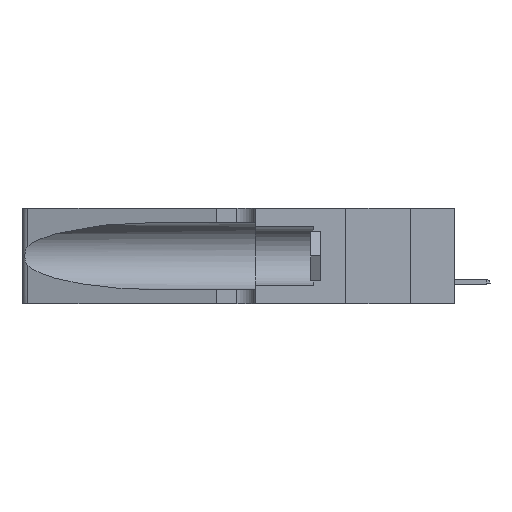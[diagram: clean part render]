
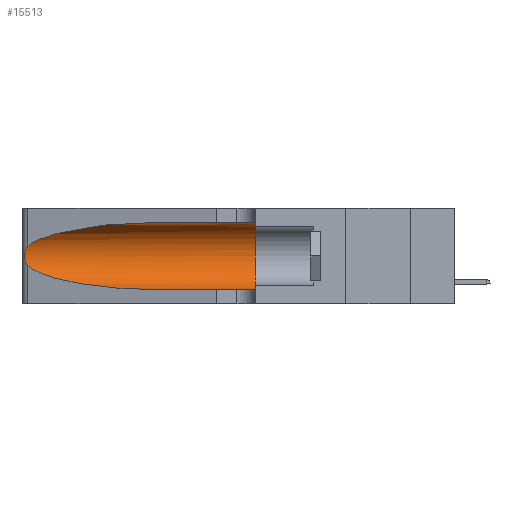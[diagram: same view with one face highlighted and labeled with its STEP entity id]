
A CAD part, left-side view. The second image highlights one B-rep face of the part: STEP entity #15513.
In plain terms, the highlighted cylindrical face has radius 3.308 mm (diameter 6.617 mm), a partial arc.
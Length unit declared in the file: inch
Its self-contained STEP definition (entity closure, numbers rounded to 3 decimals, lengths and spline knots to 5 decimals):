
#500 = CARTESIAN_POINT ( 'NONE',  ( 0.26018, 1.23835, 0.19895 ) ) ;
#1418 = VERTEX_POINT ( 'NONE', #24342 ) ;
#1615 = LINE ( 'NONE', #13818, #26982 ) ;
#2284 = EDGE_CURVE ( 'NONE', #27723, #1418, #1615, .T. ) ;
#5105 = CARTESIAN_POINT ( 'NONE',  ( 0.18966, 0.96281, 0.31525 ) ) ;
#5644 = VERTEX_POINT ( 'NONE', #38142 ) ;
#6279 = DIRECTION ( 'NONE',  ( 0., 1., 0. ) ) ;
#6294 = VERTEX_POINT ( 'NONE', #31980 ) ;
#6656 = AXIS2_PLACEMENT_3D ( 'NONE', #29112, #31883, #32481 ) ;
#7006 = CARTESIAN_POINT ( 'NONE',  ( 0.25856, 1.23593, 0.16098 ) ) ;
#7173 = DIRECTION ( 'NONE',  ( 0., -1., 0. ) ) ;
#7711 = ORIENTED_EDGE ( 'NONE', *, *, #32891, .T. ) ;
#7900 = FACE_OUTER_BOUND ( 'NONE', #38821, .T. ) ;
#8730 = CARTESIAN_POINT ( 'NONE',  ( 0.25487, 1.22718, 0.14631 ) ) ;
#9931 = CARTESIAN_POINT ( 'NONE',  ( 0.26017, 1.23833, 0.17102 ) ) ;
#10299 = CARTESIAN_POINT ( 'NONE',  ( 0.1305, 1.61858, 0.05475 ) ) ;
#11039 = CARTESIAN_POINT ( 'NONE',  ( 0.1305, 0.72297, 0.31525 ) ) ;
#11617 = CARTESIAN_POINT ( 'NONE',  ( 0.1305, 0.72297, 0.05475 ) ) ;
#12183 = CARTESIAN_POINT ( 'NONE',  ( 0.1305, 0.35, 0.185 ) ) ;
#12521 = CARTESIAN_POINT ( 'NONE',  ( 0.25555, 1.22993, 0.14849 ) ) ;
#12930 = EDGE_CURVE ( 'NONE', #1418, #5644, #25940, .T. ) ;
#13389 = CARTESIAN_POINT ( 'NONE',  ( 0.1305, 0.72297, 0.05475 ) ) ;
#13818 = CARTESIAN_POINT ( 'NONE',  ( 0.1305, 1.61858, 0.31525 ) ) ;
#14164 = CARTESIAN_POINT ( 'NONE',  ( 0.2373, 1.15595, 0.28018 ) ) ;
#15513 = ADVANCED_FACE ( 'NONE', ( #7900 ), #32087, .F. ) ;
#16052 = CARTESIAN_POINT ( 'NONE',  ( 0.25639, 1.23186, 0.15144 ) ) ;
#17863 = VECTOR ( 'NONE', #7173, 39.37008 ) ;
#18052 = EDGE_CURVE ( 'NONE', #6294, #21579, #19097, .T. ) ;
#18877 = CARTESIAN_POINT ( 'NONE',  ( 0.25487, 1.22718, 0.14631 ) ) ;
#18974 = CARTESIAN_POINT ( 'NONE',  ( 0.26075, 1.23896, 0.19203 ) ) ;
#19097 = B_SPLINE_CURVE_WITH_KNOTS ( 'NONE', 3,
 ( #31183, #24871, #24491, #30425, #36910, #500, #18974, #33961, #9931, #7006, #30990, #16052, #12521, #8730 ),
 .UNSPECIFIED., .F., .F.,
 ( 4, 2, 2, 2, 2, 2, 4 ),
 ( 0., 0.00027, 0.00053, 0.00107, 0.0016, 0.00187, 0.00214 ),
 .UNSPECIFIED. ) ;
#19181 = ORIENTED_EDGE ( 'NONE', *, *, #31482, .T. ) ;
#19891 = DIRECTION ( 'NONE',  ( 0., -1., 0. ) ) ;
#19926 = ORIENTED_EDGE ( 'NONE', *, *, #37539, .T. ) ;
#20940 =( BOUNDED_CURVE ( )  B_SPLINE_CURVE ( 3, ( #18877, #30886, #30695, #13389 ),
 .UNSPECIFIED., .F., .T. ) 
 B_SPLINE_CURVE_WITH_KNOTS ( ( 4, 4 ),
 ( 3.44316, 4.71239 ),
 .UNSPECIFIED. ) 
 CURVE ( )  GEOMETRIC_REPRESENTATION_ITEM ( )  RATIONAL_B_SPLINE_CURVE ( ( 1., 0.87, 0.87, 1. ) ) 
 REPRESENTATION_ITEM ( '' )  );
#21579 = VERTEX_POINT ( 'NONE', #32590 ) ;
#21766 = ORIENTED_EDGE ( 'NONE', *, *, #12930, .F. ) ;
#24342 = CARTESIAN_POINT ( 'NONE',  ( 0.1305, 0.35, 0.31525 ) ) ;
#24491 = CARTESIAN_POINT ( 'NONE',  ( 0.25639, 1.23184, 0.21858 ) ) ;
#24871 = CARTESIAN_POINT ( 'NONE',  ( 0.25555, 1.22994, 0.2215 ) ) ;
#24913 = DIRECTION ( 'NONE',  ( 0., 0., 1. ) ) ;
#24956 =( BOUNDED_CURVE ( )  B_SPLINE_CURVE ( 3, ( #28896, #5105, #14164, #38382 ),
 .UNSPECIFIED., .F., .F. ) 
 B_SPLINE_CURVE_WITH_KNOTS ( ( 4, 4 ),
 ( 1.5708, 2.84003 ),
 .UNSPECIFIED. ) 
 CURVE ( )  GEOMETRIC_REPRESENTATION_ITEM ( )  RATIONAL_B_SPLINE_CURVE ( ( 1., 0.87, 0.87, 1. ) ) 
 REPRESENTATION_ITEM ( '' )  );
#25609 = LINE ( 'NONE', #10299, #17863 ) ;
#25940 = CIRCLE ( 'NONE', #38585, 0.13025 ) ;
#26519 = ORIENTED_EDGE ( 'NONE', *, *, #18052, .T. ) ;
#26593 = ORIENTED_EDGE ( 'NONE', *, *, #2284, .F. ) ;
#26982 = VECTOR ( 'NONE', #19891, 39.37008 ) ;
#27723 = VERTEX_POINT ( 'NONE', #11039 ) ;
#28896 = CARTESIAN_POINT ( 'NONE',  ( 0.1305, 0.72297, 0.31525 ) ) ;
#29112 = CARTESIAN_POINT ( 'NONE',  ( 0.1305, 1.61858, 0.185 ) ) ;
#30425 = CARTESIAN_POINT ( 'NONE',  ( 0.25787, 1.23484, 0.2124 ) ) ;
#30695 = CARTESIAN_POINT ( 'NONE',  ( 0.18966, 0.96281, 0.05475 ) ) ;
#30886 = CARTESIAN_POINT ( 'NONE',  ( 0.2373, 1.15595, 0.08982 ) ) ;
#30990 = CARTESIAN_POINT ( 'NONE',  ( 0.25789, 1.23486, 0.15765 ) ) ;
#31183 = CARTESIAN_POINT ( 'NONE',  ( 0.25487, 1.22718, 0.22369 ) ) ;
#31482 = EDGE_CURVE ( 'NONE', #21579, #34091, #20940, .T. ) ;
#31883 = DIRECTION ( 'NONE',  ( 0., -1., 0. ) ) ;
#31980 = CARTESIAN_POINT ( 'NONE',  ( 0.25487, 1.22718, 0.22369 ) ) ;
#32087 = CYLINDRICAL_SURFACE ( 'NONE', #6656, 0.13025 ) ;
#32481 = DIRECTION ( 'NONE',  ( 0., 0., -1. ) ) ;
#32590 = CARTESIAN_POINT ( 'NONE',  ( 0.25487, 1.22718, 0.14631 ) ) ;
#32891 = EDGE_CURVE ( 'NONE', #27723, #6294, #24956, .T. ) ;
#33961 = CARTESIAN_POINT ( 'NONE',  ( 0.26075, 1.23896, 0.178 ) ) ;
#34091 = VERTEX_POINT ( 'NONE', #11617 ) ;
#36910 = CARTESIAN_POINT ( 'NONE',  ( 0.25854, 1.2359, 0.20912 ) ) ;
#37539 = EDGE_CURVE ( 'NONE', #34091, #5644, #25609, .T. ) ;
#38142 = CARTESIAN_POINT ( 'NONE',  ( 0.1305, 0.35, 0.05475 ) ) ;
#38382 = CARTESIAN_POINT ( 'NONE',  ( 0.25487, 1.22718, 0.22369 ) ) ;
#38585 = AXIS2_PLACEMENT_3D ( 'NONE', #12183, #6279, #24913 ) ;
#38821 = EDGE_LOOP ( 'NONE', ( #7711, #26519, #19181, #19926, #21766, #26593 ) ) ;
